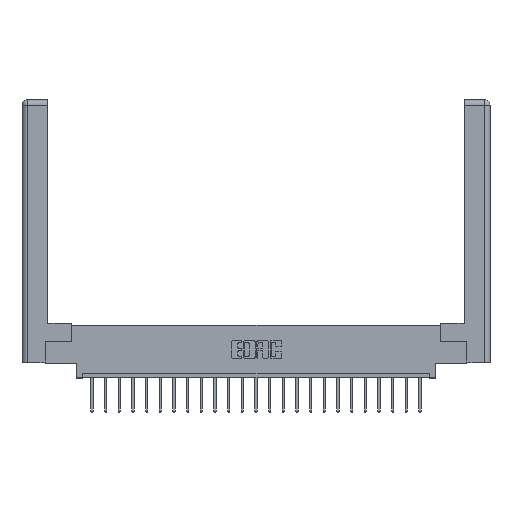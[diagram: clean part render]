
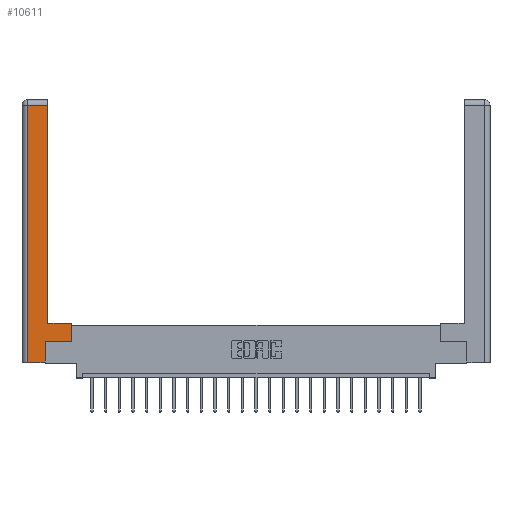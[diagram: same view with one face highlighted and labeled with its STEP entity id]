
A CAD part, top view. The second image highlights one B-rep face of the part: STEP entity #10611.
In plain terms, the highlighted planar face has unit normal (0, 0, 1).
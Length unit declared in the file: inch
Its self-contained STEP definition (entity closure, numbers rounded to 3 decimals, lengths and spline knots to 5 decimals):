
#435 = ORIENTED_EDGE ( 'NONE', *, *, #16357, .T. ) ;
#615 = VECTOR ( 'NONE', #16690, 39.37008 ) ;
#911 = EDGE_LOOP ( 'NONE', ( #15921, #15936, #7676, #435, #7911, #7990, #14187, #11142 ) ) ;
#1362 = EDGE_CURVE ( 'NONE', #6772, #20441, #4043, .T. ) ;
#1662 = EDGE_CURVE ( 'NONE', #21537, #23072, #18286, .T. ) ;
#1751 = DIRECTION ( 'NONE',  ( 0., 1., 0. ) ) ;
#2271 = CARTESIAN_POINT ( 'NONE',  ( 0.0615, 2.94, 0. ) ) ;
#2462 = EDGE_CURVE ( 'NONE', #20441, #21537, #20267, .T. ) ;
#2912 = DIRECTION ( 'NONE',  ( 1., 0., 0. ) ) ;
#3275 = VECTOR ( 'NONE', #2912, 39.37008 ) ;
#3307 = DIRECTION ( 'NONE',  ( -1., 0., 0. ) ) ;
#4043 = LINE ( 'NONE', #13971, #7723 ) ;
#4438 = AXIS2_PLACEMENT_3D ( 'NONE', #12309, #4908, #3307 ) ;
#4545 = PLANE ( 'NONE',  #4438 ) ;
#4567 = CARTESIAN_POINT ( 'NONE',  ( 0.0615, 2.94, 0. ) ) ;
#4908 = DIRECTION ( 'NONE',  ( 0., 0., -1. ) ) ;
#5222 = CARTESIAN_POINT ( 'NONE',  ( 0.565, 0.245, 0. ) ) ;
#6104 = CARTESIAN_POINT ( 'NONE',  ( 0.295, 3., 0. ) ) ;
#6221 = CARTESIAN_POINT ( 'NONE',  ( 0.295, 0.45, 0. ) ) ;
#6641 = CARTESIAN_POINT ( 'NONE',  ( 0.0615, 0., 0. ) ) ;
#6696 = VECTOR ( 'NONE', #16965, 39.37008 ) ;
#6772 = VERTEX_POINT ( 'NONE', #20973 ) ;
#7021 = DIRECTION ( 'NONE',  ( 0., 1., 0. ) ) ;
#7494 = EDGE_CURVE ( 'NONE', #7626, #12125, #8389, .T. ) ;
#7626 = VERTEX_POINT ( 'NONE', #16502 ) ;
#7676 = ORIENTED_EDGE ( 'NONE', *, *, #9217, .T. ) ;
#7723 = VECTOR ( 'NONE', #19794, 39.37008 ) ;
#7911 = ORIENTED_EDGE ( 'NONE', *, *, #7494, .T. ) ;
#7990 = ORIENTED_EDGE ( 'NONE', *, *, #13383, .T. ) ;
#8359 = DIRECTION ( 'NONE',  ( 0., -1., 0. ) ) ;
#8389 = LINE ( 'NONE', #10754, #8952 ) ;
#8952 = VECTOR ( 'NONE', #1751, 39.37008 ) ;
#9217 = EDGE_CURVE ( 'NONE', #13344, #16236, #19997, .T. ) ;
#10611 = ADVANCED_FACE ( 'NONE', ( #19383 ), #4545, .F. ) ;
#10754 = CARTESIAN_POINT ( 'NONE',  ( 0.265, 0.245, 0. ) ) ;
#11056 = CARTESIAN_POINT ( 'NONE',  ( 0.565, 0.45, 0. ) ) ;
#11142 = ORIENTED_EDGE ( 'NONE', *, *, #2462, .T. ) ;
#12125 = VERTEX_POINT ( 'NONE', #15740 ) ;
#12309 = CARTESIAN_POINT ( 'NONE',  ( 0., 0., 0. ) ) ;
#12789 = LINE ( 'NONE', #23452, #19368 ) ;
#13237 = EDGE_CURVE ( 'NONE', #23072, #13344, #18127, .T. ) ;
#13344 = VERTEX_POINT ( 'NONE', #4567 ) ;
#13383 = EDGE_CURVE ( 'NONE', #12125, #6772, #13549, .T. ) ;
#13549 = LINE ( 'NONE', #5222, #3275 ) ;
#13971 = CARTESIAN_POINT ( 'NONE',  ( 0.565, 0.45, 0. ) ) ;
#14187 = ORIENTED_EDGE ( 'NONE', *, *, #1362, .T. ) ;
#14573 = VECTOR ( 'NONE', #8359, 39.37008 ) ;
#15740 = CARTESIAN_POINT ( 'NONE',  ( 0.265, 0.245, 0. ) ) ;
#15921 = ORIENTED_EDGE ( 'NONE', *, *, #1662, .T. ) ;
#15936 = ORIENTED_EDGE ( 'NONE', *, *, #13237, .T. ) ;
#16236 = VERTEX_POINT ( 'NONE', #6641 ) ;
#16357 = EDGE_CURVE ( 'NONE', #16236, #7626, #12789, .T. ) ;
#16502 = CARTESIAN_POINT ( 'NONE',  ( 0.265, 0., 0. ) ) ;
#16690 = DIRECTION ( 'NONE',  ( -1., 0., 0. ) ) ;
#16965 = DIRECTION ( 'NONE',  ( -1., 0., 0. ) ) ;
#17426 = VECTOR ( 'NONE', #7021, 39.37008 ) ;
#18127 = LINE ( 'NONE', #2271, #6696 ) ;
#18286 = LINE ( 'NONE', #6104, #17426 ) ;
#18828 = DIRECTION ( 'NONE',  ( 1., 0., 0. ) ) ;
#19368 = VECTOR ( 'NONE', #18828, 39.37008 ) ;
#19383 = FACE_OUTER_BOUND ( 'NONE', #911, .T. ) ;
#19725 = CARTESIAN_POINT ( 'NONE',  ( 0.295, 0.45, 0. ) ) ;
#19794 = DIRECTION ( 'NONE',  ( 0., 1., 0. ) ) ;
#19997 = LINE ( 'NONE', #21195, #14573 ) ;
#20267 = LINE ( 'NONE', #19725, #615 ) ;
#20441 = VERTEX_POINT ( 'NONE', #11056 ) ;
#20973 = CARTESIAN_POINT ( 'NONE',  ( 0.565, 0.245, 0. ) ) ;
#21195 = CARTESIAN_POINT ( 'NONE',  ( 0.0615, 0., 0. ) ) ;
#21537 = VERTEX_POINT ( 'NONE', #6221 ) ;
#21881 = CARTESIAN_POINT ( 'NONE',  ( 0.295, 2.94, 0. ) ) ;
#23072 = VERTEX_POINT ( 'NONE', #21881 ) ;
#23452 = CARTESIAN_POINT ( 'NONE',  ( 0.265, 0., 0. ) ) ;
